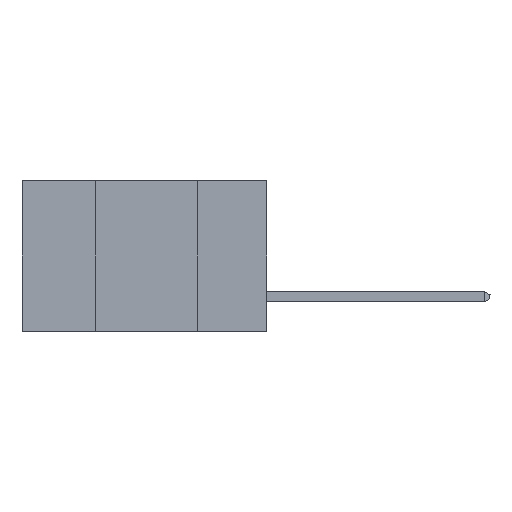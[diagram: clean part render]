
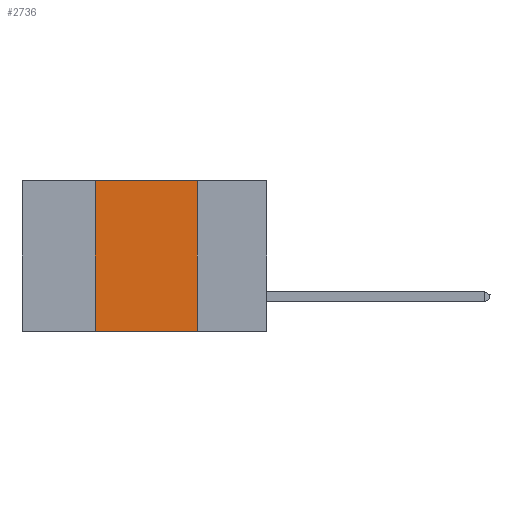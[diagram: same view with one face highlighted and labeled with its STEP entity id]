
A CAD part, left-side view. The second image highlights one B-rep face of the part: STEP entity #2736.
In plain terms, the highlighted planar face has unit normal (-1, 0, 0).
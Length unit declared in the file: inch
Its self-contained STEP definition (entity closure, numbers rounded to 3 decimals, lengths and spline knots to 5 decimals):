
#257 = VECTOR ( 'NONE', #30600, 39.37008 ) ;
#718 = ORIENTED_EDGE ( 'NONE', *, *, #13882, .F. ) ;
#1842 = DIRECTION ( 'NONE',  ( 0., 0., 1. ) ) ;
#2721 = CARTESIAN_POINT ( 'NONE',  ( 0., 0.6, 0. ) ) ;
#2736 = ADVANCED_FACE ( 'NONE', ( #2969 ), #10921, .F. ) ;
#2912 = VECTOR ( 'NONE', #1842, 39.37008 ) ;
#2969 = FACE_OUTER_BOUND ( 'NONE', #15676, .T. ) ;
#6484 = VECTOR ( 'NONE', #18625, 39.37008 ) ;
#9838 = CARTESIAN_POINT ( 'NONE',  ( 0., 0.6, -0.37 ) ) ;
#10516 = LINE ( 'NONE', #21589, #6484 ) ;
#10921 = PLANE ( 'NONE',  #29932 ) ;
#13882 = EDGE_CURVE ( 'NONE', #17807, #24561, #28033, .T. ) ;
#14380 = VERTEX_POINT ( 'NONE', #28711 ) ;
#15190 = EDGE_CURVE ( 'NONE', #25306, #17807, #33619, .T. ) ;
#15676 = EDGE_LOOP ( 'NONE', ( #23671, #718, #24816, #28517 ) ) ;
#17807 = VERTEX_POINT ( 'NONE', #24060 ) ;
#18504 = DIRECTION ( 'NONE',  ( 0., -1., 0. ) ) ;
#18625 = DIRECTION ( 'NONE',  ( 0., 0., -1. ) ) ;
#19399 = DIRECTION ( 'NONE',  ( 0., 0., -1. ) ) ;
#21589 = CARTESIAN_POINT ( 'NONE',  ( 0., 0.17, 0. ) ) ;
#22180 = CARTESIAN_POINT ( 'NONE',  ( 0., 0.6, 0. ) ) ;
#22564 = CARTESIAN_POINT ( 'NONE',  ( 0., 0.42, -0.37 ) ) ;
#23671 = ORIENTED_EDGE ( 'NONE', *, *, #32957, .F. ) ;
#24060 = CARTESIAN_POINT ( 'NONE',  ( 0., 0.42, 0. ) ) ;
#24561 = VERTEX_POINT ( 'NONE', #32401 ) ;
#24816 = ORIENTED_EDGE ( 'NONE', *, *, #15190, .F. ) ;
#25306 = VERTEX_POINT ( 'NONE', #22564 ) ;
#25957 = VECTOR ( 'NONE', #18504, 39.37008 ) ;
#28033 = LINE ( 'NONE', #2721, #257 ) ;
#28517 = ORIENTED_EDGE ( 'NONE', *, *, #34992, .T. ) ;
#28711 = CARTESIAN_POINT ( 'NONE',  ( 0., 0.17, -0.37 ) ) ;
#29932 = AXIS2_PLACEMENT_3D ( 'NONE', #22180, #33438, #19399 ) ;
#30600 = DIRECTION ( 'NONE',  ( 0., -1., 0. ) ) ;
#32401 = CARTESIAN_POINT ( 'NONE',  ( 0., 0.17, 0. ) ) ;
#32729 = LINE ( 'NONE', #9838, #25957 ) ;
#32957 = EDGE_CURVE ( 'NONE', #24561, #14380, #10516, .T. ) ;
#33058 = CARTESIAN_POINT ( 'NONE',  ( 0., 0.42, 0. ) ) ;
#33438 = DIRECTION ( 'NONE',  ( 1., 0., 0. ) ) ;
#33619 = LINE ( 'NONE', #33058, #2912 ) ;
#34992 = EDGE_CURVE ( 'NONE', #25306, #14380, #32729, .T. ) ;
